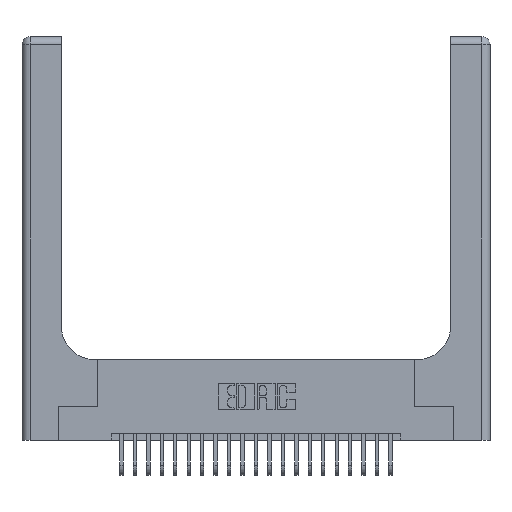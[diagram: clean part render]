
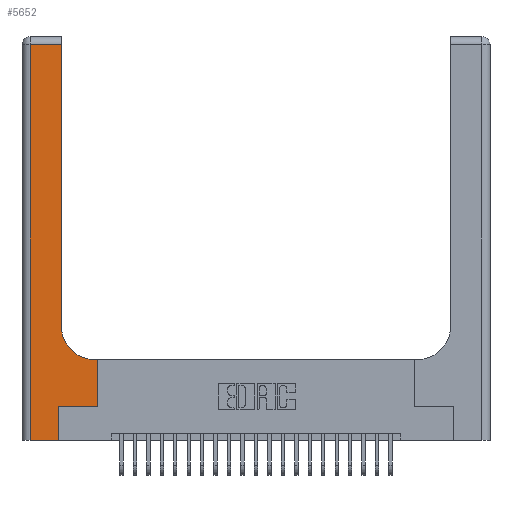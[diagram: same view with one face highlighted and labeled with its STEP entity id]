
A CAD part, top view. The second image highlights one B-rep face of the part: STEP entity #5652.
In plain terms, the highlighted planar face has unit normal (0, 0, 1).
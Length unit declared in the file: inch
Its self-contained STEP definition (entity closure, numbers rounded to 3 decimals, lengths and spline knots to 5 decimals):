
#44 = DIRECTION ( 'NONE',  ( -1., 0., 0. ) ) ;
#330 = VERTEX_POINT ( 'NONE', #4054 ) ;
#782 = EDGE_LOOP ( 'NONE', ( #3717, #9112, #22173, #12296, #12730, #5091, #19834, #13918, #9594 ) ) ;
#1294 = CARTESIAN_POINT ( 'NONE',  ( 0.06, 2.94, 0.37 ) ) ;
#1467 = VERTEX_POINT ( 'NONE', #23537 ) ;
#1546 = DIRECTION ( 'NONE',  ( 1., 0., 0. ) ) ;
#2223 = EDGE_CURVE ( 'NONE', #21590, #23189, #7048, .T. ) ;
#2514 = AXIS2_PLACEMENT_3D ( 'NONE', #21114, #10221, #22897 ) ;
#3082 = CARTESIAN_POINT ( 'NONE',  ( 0.269, 0., 0.37 ) ) ;
#3529 = DIRECTION ( 'NONE',  ( 1., 0., 0. ) ) ;
#3717 = ORIENTED_EDGE ( 'NONE', *, *, #18142, .T. ) ;
#3831 = CARTESIAN_POINT ( 'NONE',  ( 0.06, 3., 0.37 ) ) ;
#4054 = CARTESIAN_POINT ( 'NONE',  ( 0.5585, 0.25, 0.37 ) ) ;
#4891 = VERTEX_POINT ( 'NONE', #17984 ) ;
#4895 = EDGE_CURVE ( 'NONE', #22292, #330, #23740, .T. ) ;
#5091 = ORIENTED_EDGE ( 'NONE', *, *, #4895, .T. ) ;
#5399 = CARTESIAN_POINT ( 'NONE',  ( 0.269, 0.25, 0.37 ) ) ;
#5652 = ADVANCED_FACE ( 'NONE', ( #7143 ), #11465, .F. ) ;
#5668 = VERTEX_POINT ( 'NONE', #17020 ) ;
#6165 = EDGE_CURVE ( 'NONE', #14972, #16721, #16355, .T. ) ;
#6644 = EDGE_CURVE ( 'NONE', #23189, #5668, #17462, .T. ) ;
#7048 = LINE ( 'NONE', #22183, #21074 ) ;
#7085 = CARTESIAN_POINT ( 'NONE',  ( 0.5585, 0.6, 0.37 ) ) ;
#7122 = VECTOR ( 'NONE', #16835, 39.37008 ) ;
#7143 = FACE_OUTER_BOUND ( 'NONE', #782, .T. ) ;
#7674 = LINE ( 'NONE', #3082, #16898 ) ;
#8684 = CARTESIAN_POINT ( 'NONE',  ( 0.06, 0., 0.37 ) ) ;
#9112 = ORIENTED_EDGE ( 'NONE', *, *, #20920, .T. ) ;
#9594 = ORIENTED_EDGE ( 'NONE', *, *, #6644, .T. ) ;
#9635 = CARTESIAN_POINT ( 'NONE',  ( 0., 3., 0.37 ) ) ;
#9785 = CARTESIAN_POINT ( 'NONE',  ( 0.5415, 0.6, 0.37 ) ) ;
#9960 = VECTOR ( 'NONE', #11973, 39.37008 ) ;
#10067 = CARTESIAN_POINT ( 'NONE',  ( 0.2915, 3., 0.37 ) ) ;
#10221 = DIRECTION ( 'NONE',  ( 0., 0., -1. ) ) ;
#10390 = CARTESIAN_POINT ( 'NONE',  ( 0., 2.94, 0.37 ) ) ;
#11043 = LINE ( 'NONE', #10390, #15319 ) ;
#11320 = DIRECTION ( 'NONE',  ( 0., 1., 0. ) ) ;
#11465 = PLANE ( 'NONE',  #16414 ) ;
#11546 = DIRECTION ( 'NONE',  ( -1., 0., 0. ) ) ;
#11825 = EDGE_CURVE ( 'NONE', #330, #21590, #21602, .T. ) ;
#11973 = DIRECTION ( 'NONE',  ( 0., 1., 0. ) ) ;
#12012 = VECTOR ( 'NONE', #11320, 39.37008 ) ;
#12296 = ORIENTED_EDGE ( 'NONE', *, *, #18466, .T. ) ;
#12300 = VECTOR ( 'NONE', #3529, 39.37008 ) ;
#12730 = ORIENTED_EDGE ( 'NONE', *, *, #16077, .T. ) ;
#13918 = ORIENTED_EDGE ( 'NONE', *, *, #2223, .T. ) ;
#14291 = DIRECTION ( 'NONE',  ( 0., 1., 0. ) ) ;
#14721 = CARTESIAN_POINT ( 'NONE',  ( 0., 0., 0.37 ) ) ;
#14863 = LINE ( 'NONE', #10067, #9960 ) ;
#14972 = VERTEX_POINT ( 'NONE', #1294 ) ;
#14985 = CARTESIAN_POINT ( 'NONE',  ( 0.269, 0.25, 0.37 ) ) ;
#15319 = VECTOR ( 'NONE', #15912, 39.37008 ) ;
#15912 = DIRECTION ( 'NONE',  ( -1., 0., 0. ) ) ;
#16077 = EDGE_CURVE ( 'NONE', #4891, #22292, #7674, .T. ) ;
#16355 = LINE ( 'NONE', #3831, #7122 ) ;
#16414 = AXIS2_PLACEMENT_3D ( 'NONE', #9635, #22347, #11546 ) ;
#16721 = VERTEX_POINT ( 'NONE', #8684 ) ;
#16728 = CARTESIAN_POINT ( 'NONE',  ( 0.5585, 0.25, 0.37 ) ) ;
#16835 = DIRECTION ( 'NONE',  ( 0., -1., 0. ) ) ;
#16898 = VECTOR ( 'NONE', #14291, 39.37008 ) ;
#17020 = CARTESIAN_POINT ( 'NONE',  ( 0.2915, 0.85, 0.37 ) ) ;
#17462 = CIRCLE ( 'NONE', #2514, 0.25 ) ;
#17984 = CARTESIAN_POINT ( 'NONE',  ( 0.269, 0., 0.37 ) ) ;
#18142 = EDGE_CURVE ( 'NONE', #5668, #1467, #14863, .T. ) ;
#18466 = EDGE_CURVE ( 'NONE', #16721, #4891, #22440, .T. ) ;
#18960 = VECTOR ( 'NONE', #1546, 39.37008 ) ;
#19834 = ORIENTED_EDGE ( 'NONE', *, *, #11825, .T. ) ;
#20920 = EDGE_CURVE ( 'NONE', #1467, #14972, #11043, .T. ) ;
#21074 = VECTOR ( 'NONE', #44, 39.37008 ) ;
#21114 = CARTESIAN_POINT ( 'NONE',  ( 0.5415, 0.85, 0.37 ) ) ;
#21590 = VERTEX_POINT ( 'NONE', #7085 ) ;
#21602 = LINE ( 'NONE', #16728, #12012 ) ;
#22173 = ORIENTED_EDGE ( 'NONE', *, *, #6165, .T. ) ;
#22183 = CARTESIAN_POINT ( 'NONE',  ( 0.2915, 0.6, 0.37 ) ) ;
#22292 = VERTEX_POINT ( 'NONE', #14985 ) ;
#22347 = DIRECTION ( 'NONE',  ( 0., 0., -1. ) ) ;
#22440 = LINE ( 'NONE', #14721, #12300 ) ;
#22897 = DIRECTION ( 'NONE',  ( 1., 0., 0. ) ) ;
#23189 = VERTEX_POINT ( 'NONE', #9785 ) ;
#23537 = CARTESIAN_POINT ( 'NONE',  ( 0.2915, 2.94, 0.37 ) ) ;
#23740 = LINE ( 'NONE', #5399, #18960 ) ;
